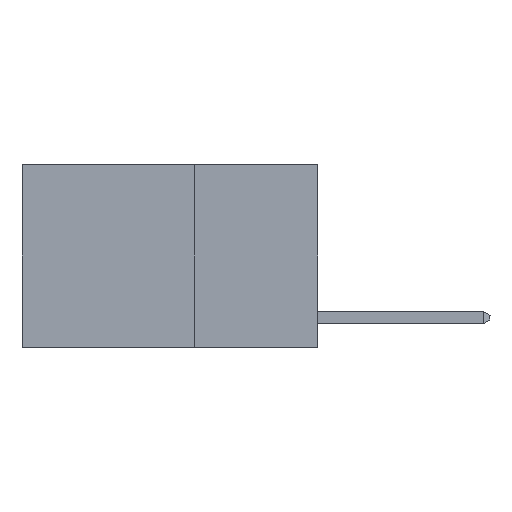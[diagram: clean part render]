
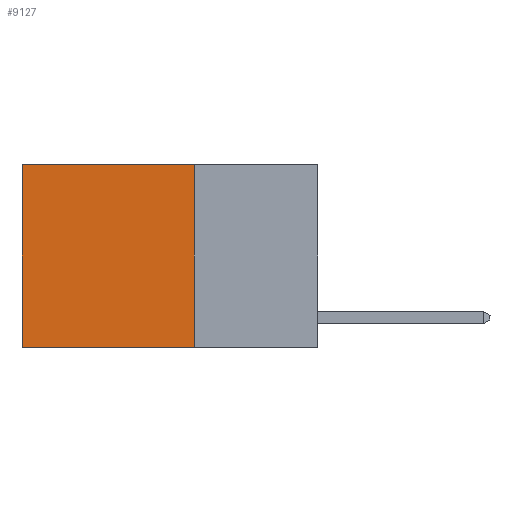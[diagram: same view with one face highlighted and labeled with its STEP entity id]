
A CAD part, left-side view. The second image highlights one B-rep face of the part: STEP entity #9127.
In plain terms, the highlighted planar face has unit normal (-1, 0, 0).
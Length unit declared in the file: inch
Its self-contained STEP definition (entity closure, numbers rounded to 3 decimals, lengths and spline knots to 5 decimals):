
#592 = VERTEX_POINT ( 'NONE', #6755 ) ;
#641 = EDGE_CURVE ( 'NONE', #9573, #592, #16314, .T. ) ;
#774 = DIRECTION ( 'NONE',  ( 1., 0., 0. ) ) ;
#799 = CARTESIAN_POINT ( 'NONE',  ( 0.2625, 0.6, -0.37 ) ) ;
#1274 = ORIENTED_EDGE ( 'NONE', *, *, #641, .F. ) ;
#1430 = VERTEX_POINT ( 'NONE', #4879 ) ;
#1816 = FACE_OUTER_BOUND ( 'NONE', #7629, .T. ) ;
#4298 = LINE ( 'NONE', #14786, #11423 ) ;
#4318 = LINE ( 'NONE', #12265, #7515 ) ;
#4508 = CARTESIAN_POINT ( 'NONE',  ( 0.2625, 0.25, 0. ) ) ;
#4879 = CARTESIAN_POINT ( 'NONE',  ( 0.2625, 0.6, 0. ) ) ;
#5228 = LINE ( 'NONE', #14617, #11911 ) ;
#6552 = DIRECTION ( 'NONE',  ( 0., 0., -1. ) ) ;
#6572 = ORIENTED_EDGE ( 'NONE', *, *, #17229, .T. ) ;
#6755 = CARTESIAN_POINT ( 'NONE',  ( 0.2625, 0.25, -0.37 ) ) ;
#7515 = VECTOR ( 'NONE', #14919, 39.37008 ) ;
#7629 = EDGE_LOOP ( 'NONE', ( #8803, #15543, #1274, #6572 ) ) ;
#7676 = AXIS2_PLACEMENT_3D ( 'NONE', #8952, #774, #10260 ) ;
#8528 = VERTEX_POINT ( 'NONE', #799 ) ;
#8803 = ORIENTED_EDGE ( 'NONE', *, *, #16800, .T. ) ;
#8952 = CARTESIAN_POINT ( 'NONE',  ( 0.2625, 0.25, 0. ) ) ;
#9127 = ADVANCED_FACE ( 'NONE', ( #1816 ), #16811, .F. ) ;
#9297 = DIRECTION ( 'NONE',  ( 0., 1., 0. ) ) ;
#9573 = VERTEX_POINT ( 'NONE', #4508 ) ;
#10260 = DIRECTION ( 'NONE',  ( 0., 0., -1. ) ) ;
#11423 = VECTOR ( 'NONE', #16079, 39.37008 ) ;
#11911 = VECTOR ( 'NONE', #9297, 39.37008 ) ;
#12265 = CARTESIAN_POINT ( 'NONE',  ( 0.2625, 0.6, 0. ) ) ;
#13114 = EDGE_CURVE ( 'NONE', #592, #8528, #5228, .T. ) ;
#14617 = CARTESIAN_POINT ( 'NONE',  ( 0.2625, 0.25, -0.37 ) ) ;
#14786 = CARTESIAN_POINT ( 'NONE',  ( 0.2625, 0.25, 0. ) ) ;
#14919 = DIRECTION ( 'NONE',  ( 0., 0., -1. ) ) ;
#15543 = ORIENTED_EDGE ( 'NONE', *, *, #13114, .F. ) ;
#15915 = VECTOR ( 'NONE', #6552, 39.37008 ) ;
#16079 = DIRECTION ( 'NONE',  ( 0., 1., 0. ) ) ;
#16314 = LINE ( 'NONE', #16437, #15915 ) ;
#16437 = CARTESIAN_POINT ( 'NONE',  ( 0.2625, 0.25, 0. ) ) ;
#16800 = EDGE_CURVE ( 'NONE', #1430, #8528, #4318, .T. ) ;
#16811 = PLANE ( 'NONE',  #7676 ) ;
#17229 = EDGE_CURVE ( 'NONE', #9573, #1430, #4298, .T. ) ;
